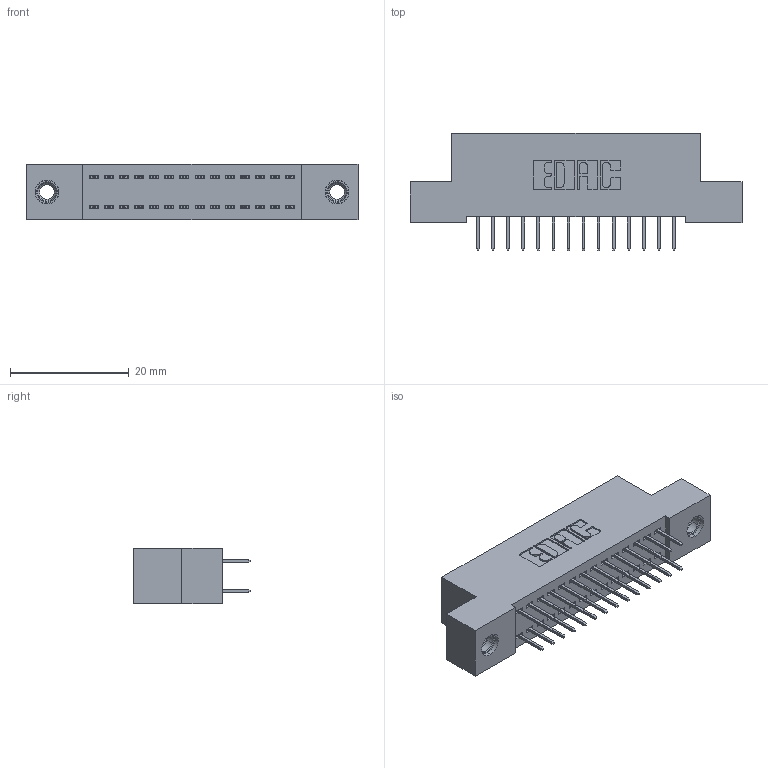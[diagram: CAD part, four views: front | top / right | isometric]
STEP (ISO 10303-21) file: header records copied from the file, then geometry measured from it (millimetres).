
FILE_DESCRIPTION (( 'STEP AP203' ), '1' );
FILE_NAME ('392-028-524-207.STEP', '2018-08-15T20:59:53', ( '' ), ( '' ), 'SwSTEP 2.0', 'SolidWorks 2016', '' );
FILE_SCHEMA (( 'CONFIG_CONTROL_DESIGN' ));
Length unit declared in the file: inch
Products named in the file (4): 342 Part_TI; 345-292-001_345-293-124; 345-250-001_345-250-005-103; 392-028-524-207
Assembly tree (31 placements, depth 2):
  392-028-524-207
    342 Part_TI
    345-292-001_345-293-124  x28
    345-250-001_345-250-005-103  x2
Bounding box: 55.88 x 19.69 x 9.4 mm (x, y, z)
Volume: 4833.2 mm3; surface area: 7092.9 mm2
Topology: 31 solids, 31 shells, 1738 faces, 4887 edges, 3138 vertices
Faces by surface type: plane 1274, cylinder 448, cone 12, torus 4
Entity records: 13756 total; most frequent: CARTESIAN_POINT 2293, ORIENTED_EDGE 2222, DIRECTION 2041, EDGE_CURVE 1111, LINE 967, VECTOR 967, VERTEX_POINT 732, AXIS2_PLACEMENT_3D 537
